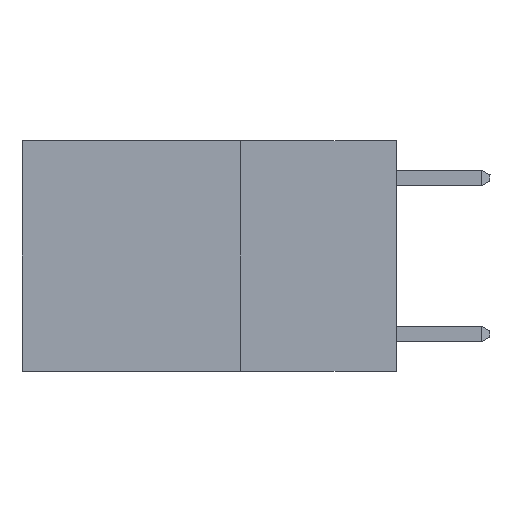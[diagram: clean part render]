
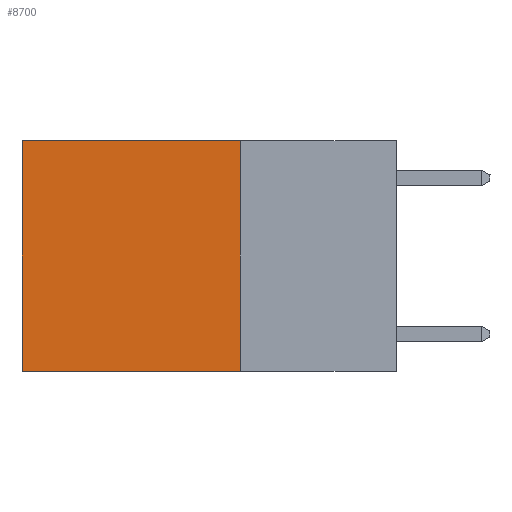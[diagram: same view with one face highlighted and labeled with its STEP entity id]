
A CAD part, left-side view. The second image highlights one B-rep face of the part: STEP entity #8700.
In plain terms, the highlighted planar face has unit normal (-1, 0, 0).
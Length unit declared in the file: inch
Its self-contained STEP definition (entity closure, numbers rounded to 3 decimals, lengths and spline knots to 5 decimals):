
#537 = CARTESIAN_POINT ( 'NONE',  ( 0.2625, 0.25, -0.37 ) ) ;
#1000 = LINE ( 'NONE', #8097, #2398 ) ;
#1153 = CARTESIAN_POINT ( 'NONE',  ( 0.2625, 0.25, 0. ) ) ;
#1216 = EDGE_CURVE ( 'NONE', #2918, #2719, #5286, .T. ) ;
#1324 = VERTEX_POINT ( 'NONE', #537 ) ;
#1404 = CARTESIAN_POINT ( 'NONE',  ( 0.2625, 0.25, 0. ) ) ;
#1717 = CARTESIAN_POINT ( 'NONE',  ( 0.2625, 0.6, 0. ) ) ;
#1744 = DIRECTION ( 'NONE',  ( 0., 0., -1. ) ) ;
#1833 = PLANE ( 'NONE',  #2688 ) ;
#2074 = DIRECTION ( 'NONE',  ( 0., 0., -1. ) ) ;
#2398 = VECTOR ( 'NONE', #8662, 39.37008 ) ;
#2513 = DIRECTION ( 'NONE',  ( 0., 0., -1. ) ) ;
#2688 = AXIS2_PLACEMENT_3D ( 'NONE', #7329, #6741, #2513 ) ;
#2719 = VERTEX_POINT ( 'NONE', #6314 ) ;
#2772 = ORIENTED_EDGE ( 'NONE', *, *, #1216, .T. ) ;
#2918 = VERTEX_POINT ( 'NONE', #1717 ) ;
#3107 = VERTEX_POINT ( 'NONE', #1153 ) ;
#3141 = CARTESIAN_POINT ( 'NONE',  ( 0.2625, 0.6, 0. ) ) ;
#3198 = ORIENTED_EDGE ( 'NONE', *, *, #4745, .F. ) ;
#3300 = LINE ( 'NONE', #7852, #5013 ) ;
#3308 = ORIENTED_EDGE ( 'NONE', *, *, #7237, .F. ) ;
#3310 = ORIENTED_EDGE ( 'NONE', *, *, #3741, .T. ) ;
#3741 = EDGE_CURVE ( 'NONE', #3107, #2918, #3300, .T. ) ;
#3811 = VECTOR ( 'NONE', #1744, 39.37008 ) ;
#3832 = DIRECTION ( 'NONE',  ( 0., 1., 0. ) ) ;
#4745 = EDGE_CURVE ( 'NONE', #1324, #2719, #1000, .T. ) ;
#5013 = VECTOR ( 'NONE', #3832, 39.37008 ) ;
#5056 = FACE_OUTER_BOUND ( 'NONE', #5688, .T. ) ;
#5286 = LINE ( 'NONE', #3141, #3811 ) ;
#5688 = EDGE_LOOP ( 'NONE', ( #2772, #3198, #3308, #3310 ) ) ;
#5867 = LINE ( 'NONE', #1404, #7340 ) ;
#6314 = CARTESIAN_POINT ( 'NONE',  ( 0.2625, 0.6, -0.37 ) ) ;
#6741 = DIRECTION ( 'NONE',  ( 1., 0., 0. ) ) ;
#7237 = EDGE_CURVE ( 'NONE', #3107, #1324, #5867, .T. ) ;
#7329 = CARTESIAN_POINT ( 'NONE',  ( 0.2625, 0.25, 0. ) ) ;
#7340 = VECTOR ( 'NONE', #2074, 39.37008 ) ;
#7852 = CARTESIAN_POINT ( 'NONE',  ( 0.2625, 0.25, 0. ) ) ;
#8097 = CARTESIAN_POINT ( 'NONE',  ( 0.2625, 0.25, -0.37 ) ) ;
#8662 = DIRECTION ( 'NONE',  ( 0., 1., 0. ) ) ;
#8700 = ADVANCED_FACE ( 'NONE', ( #5056 ), #1833, .F. ) ;
